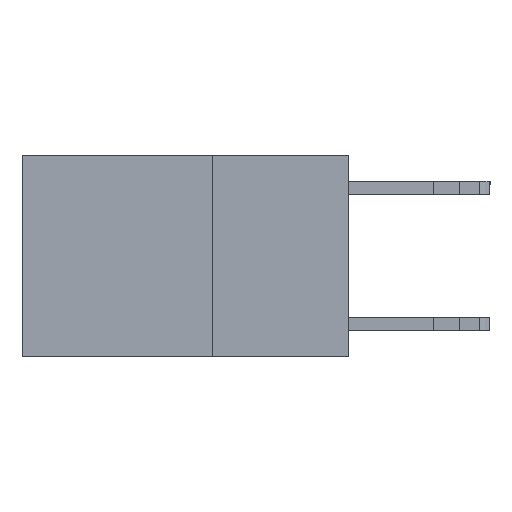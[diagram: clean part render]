
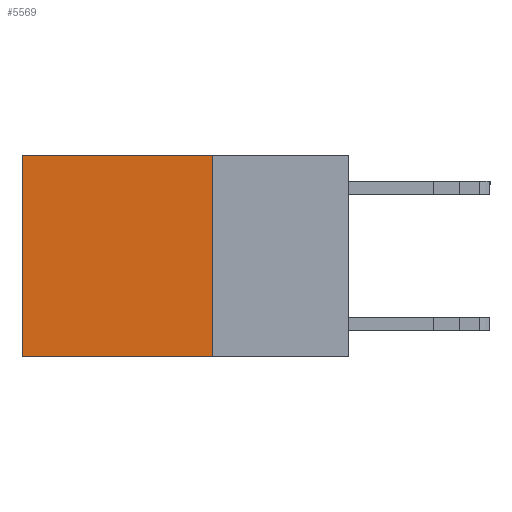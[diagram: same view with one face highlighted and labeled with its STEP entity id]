
A CAD part, left-side view. The second image highlights one B-rep face of the part: STEP entity #5569.
In plain terms, the highlighted planar face has unit normal (-1, 0, 0).
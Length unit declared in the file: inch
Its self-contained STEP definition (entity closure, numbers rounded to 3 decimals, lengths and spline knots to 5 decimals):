
#124 = VERTEX_POINT ( 'NONE', #5293 ) ;
#872 = DIRECTION ( 'NONE',  ( 1., 0., 0. ) ) ;
#1171 = VERTEX_POINT ( 'NONE', #9181 ) ;
#2202 = VECTOR ( 'NONE', #16783, 39.37008 ) ;
#2259 = EDGE_CURVE ( 'NONE', #1171, #17868, #6382, .T. ) ;
#3001 = DIRECTION ( 'NONE',  ( 0., 1., 0. ) ) ;
#4032 = DIRECTION ( 'NONE',  ( 0., 1., 0. ) ) ;
#4358 = PLANE ( 'NONE',  #5376 ) ;
#5152 = DIRECTION ( 'NONE',  ( 0., 0., -1. ) ) ;
#5293 = CARTESIAN_POINT ( 'NONE',  ( 0.2625, 0.25, 0. ) ) ;
#5376 = AXIS2_PLACEMENT_3D ( 'NONE', #16574, #872, #10584 ) ;
#5569 = ADVANCED_FACE ( 'NONE', ( #18175 ), #4358, .F. ) ;
#6361 = EDGE_CURVE ( 'NONE', #13042, #17868, #12682, .T. ) ;
#6382 = LINE ( 'NONE', #15529, #11922 ) ;
#6659 = ORIENTED_EDGE ( 'NONE', *, *, #9890, .F. ) ;
#9181 = CARTESIAN_POINT ( 'NONE',  ( 0.2625, 0.25, -0.37 ) ) ;
#9890 = EDGE_CURVE ( 'NONE', #124, #1171, #19921, .T. ) ;
#10584 = DIRECTION ( 'NONE',  ( 0., 0., -1. ) ) ;
#10598 = CARTESIAN_POINT ( 'NONE',  ( 0.2625, 0.25, 0. ) ) ;
#11180 = ORIENTED_EDGE ( 'NONE', *, *, #2259, .F. ) ;
#11922 = VECTOR ( 'NONE', #3001, 39.37008 ) ;
#11985 = CARTESIAN_POINT ( 'NONE',  ( 0.2625, 0.25, 0. ) ) ;
#12682 = LINE ( 'NONE', #19066, #17761 ) ;
#13042 = VERTEX_POINT ( 'NONE', #15074 ) ;
#13808 = VECTOR ( 'NONE', #4032, 39.37008 ) ;
#14907 = ORIENTED_EDGE ( 'NONE', *, *, #15330, .T. ) ;
#15074 = CARTESIAN_POINT ( 'NONE',  ( 0.2625, 0.6, 0. ) ) ;
#15092 = ORIENTED_EDGE ( 'NONE', *, *, #6361, .T. ) ;
#15330 = EDGE_CURVE ( 'NONE', #124, #13042, #16653, .T. ) ;
#15529 = CARTESIAN_POINT ( 'NONE',  ( 0.2625, 0.25, -0.37 ) ) ;
#16504 = CARTESIAN_POINT ( 'NONE',  ( 0.2625, 0.6, -0.37 ) ) ;
#16574 = CARTESIAN_POINT ( 'NONE',  ( 0.2625, 0.25, 0. ) ) ;
#16653 = LINE ( 'NONE', #11985, #13808 ) ;
#16783 = DIRECTION ( 'NONE',  ( 0., 0., -1. ) ) ;
#17761 = VECTOR ( 'NONE', #5152, 39.37008 ) ;
#17868 = VERTEX_POINT ( 'NONE', #16504 ) ;
#18175 = FACE_OUTER_BOUND ( 'NONE', #19611, .T. ) ;
#19066 = CARTESIAN_POINT ( 'NONE',  ( 0.2625, 0.6, 0. ) ) ;
#19611 = EDGE_LOOP ( 'NONE', ( #15092, #11180, #6659, #14907 ) ) ;
#19921 = LINE ( 'NONE', #10598, #2202 ) ;
